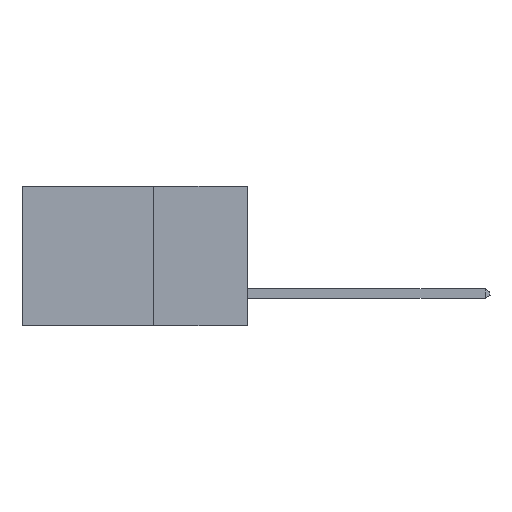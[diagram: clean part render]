
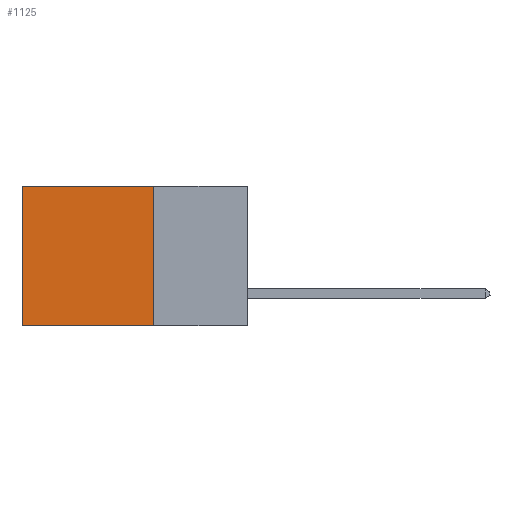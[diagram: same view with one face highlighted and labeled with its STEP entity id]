
A CAD part, left-side view. The second image highlights one B-rep face of the part: STEP entity #1125.
In plain terms, the highlighted planar face has unit normal (-1, 0, 0).
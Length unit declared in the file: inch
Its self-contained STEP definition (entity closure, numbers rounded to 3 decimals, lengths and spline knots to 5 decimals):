
#1125 = ADVANCED_FACE ( 'NONE', ( #4072 ), #7096, .F. ) ;
#1159 = VECTOR ( 'NONE', #7582, 39.37008 ) ;
#1273 = EDGE_CURVE ( 'NONE', #2986, #2187, #7492, .T. ) ;
#1557 = VERTEX_POINT ( 'NONE', #5563 ) ;
#1668 = CARTESIAN_POINT ( 'NONE',  ( 0.298, 0.25, 0. ) ) ;
#2187 = VERTEX_POINT ( 'NONE', #10885 ) ;
#2379 = DIRECTION ( 'NONE',  ( 0., 0., -1. ) ) ;
#2557 = VECTOR ( 'NONE', #2379, 39.37008 ) ;
#2986 = VERTEX_POINT ( 'NONE', #7607 ) ;
#3372 = LINE ( 'NONE', #4988, #9472 ) ;
#3710 = ORIENTED_EDGE ( 'NONE', *, *, #8817, .T. ) ;
#3863 = CARTESIAN_POINT ( 'NONE',  ( 0.298, 0.6, 0. ) ) ;
#4038 = CARTESIAN_POINT ( 'NONE',  ( 0.298, 0.25, 0. ) ) ;
#4072 = FACE_OUTER_BOUND ( 'NONE', #9132, .T. ) ;
#4384 = AXIS2_PLACEMENT_3D ( 'NONE', #7882, #10389, #4624 ) ;
#4624 = DIRECTION ( 'NONE',  ( 0., 0., -1. ) ) ;
#4988 = CARTESIAN_POINT ( 'NONE',  ( 0.298, 0.25, -0.37 ) ) ;
#5386 = ORIENTED_EDGE ( 'NONE', *, *, #1273, .F. ) ;
#5557 = ORIENTED_EDGE ( 'NONE', *, *, #9060, .F. ) ;
#5563 = CARTESIAN_POINT ( 'NONE',  ( 0.298, 0.6, 0. ) ) ;
#6889 = VERTEX_POINT ( 'NONE', #9715 ) ;
#7096 = PLANE ( 'NONE',  #4384 ) ;
#7492 = LINE ( 'NONE', #1668, #1159 ) ;
#7582 = DIRECTION ( 'NONE',  ( 0., 0., -1. ) ) ;
#7607 = CARTESIAN_POINT ( 'NONE',  ( 0.298, 0.25, 0. ) ) ;
#7709 = DIRECTION ( 'NONE',  ( 0., 1., 0. ) ) ;
#7882 = CARTESIAN_POINT ( 'NONE',  ( 0.298, 0.25, 0. ) ) ;
#8817 = EDGE_CURVE ( 'NONE', #2986, #1557, #10166, .T. ) ;
#8916 = ORIENTED_EDGE ( 'NONE', *, *, #10251, .T. ) ;
#9060 = EDGE_CURVE ( 'NONE', #2187, #6889, #3372, .T. ) ;
#9132 = EDGE_LOOP ( 'NONE', ( #8916, #5557, #5386, #3710 ) ) ;
#9298 = LINE ( 'NONE', #3863, #2557 ) ;
#9472 = VECTOR ( 'NONE', #10834, 39.37008 ) ;
#9715 = CARTESIAN_POINT ( 'NONE',  ( 0.298, 0.6, -0.37 ) ) ;
#10166 = LINE ( 'NONE', #4038, #10425 ) ;
#10251 = EDGE_CURVE ( 'NONE', #1557, #6889, #9298, .T. ) ;
#10389 = DIRECTION ( 'NONE',  ( 1., 0., 0. ) ) ;
#10425 = VECTOR ( 'NONE', #7709, 39.37008 ) ;
#10834 = DIRECTION ( 'NONE',  ( 0., 1., 0. ) ) ;
#10885 = CARTESIAN_POINT ( 'NONE',  ( 0.298, 0.25, -0.37 ) ) ;
